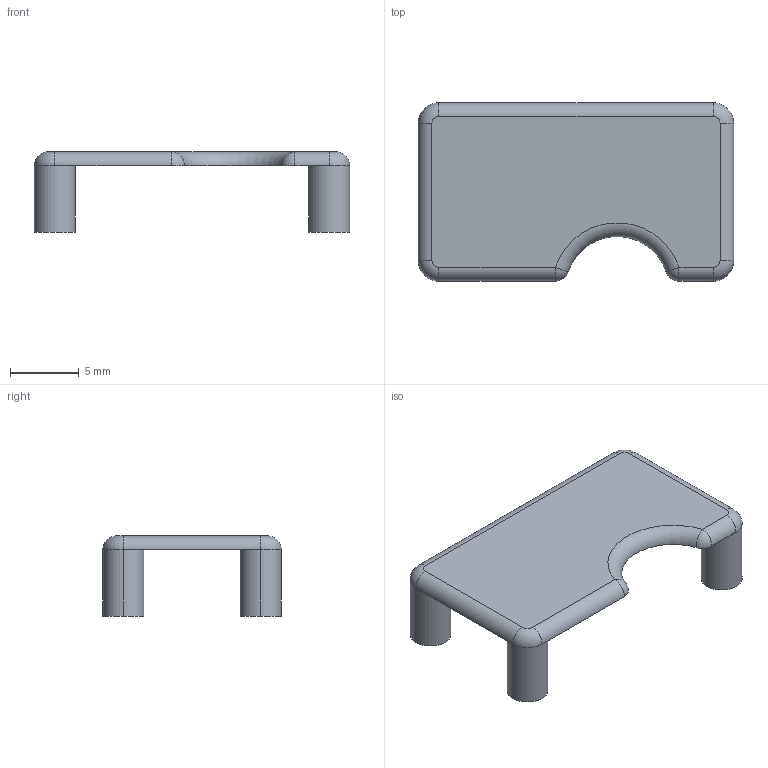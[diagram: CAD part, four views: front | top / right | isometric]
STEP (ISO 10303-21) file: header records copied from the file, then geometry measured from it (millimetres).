
FILE_DESCRIPTION (( 'STEP AP214' ), '1' );
FILE_NAME ('Mag_Release_Cover.step', '2014-05-14T06:09:11', ( 'WarFairy' ), ( '' ), 'SwSTEP 2.0', 'SolidWorks 2013', '' );
FILE_SCHEMA (( 'AUTOMOTIVE_DESIGN' ));
Length unit declared in the file: inch
Products named in the file (1): Mag_Release_Cover
Bounding box: 23 x 13 x 5.85 mm (x, y, z)
Volume: 366.1 mm3; surface area: 734.9 mm2
Topology: 1 solids, 1 shells, 23 faces, 54 edges, 31 vertices
Faces by surface type: cylinder 11, plane 5, torus 5, sphere 2
Entity records: 694 total; most frequent: DIRECTION 136, CARTESIAN_POINT 107, ORIENTED_EDGE 104, AXIS2_PLACEMENT_3D 60, EDGE_CURVE 52, CIRCLE 36, VERTEX_POINT 31, ADVANCED_FACE 23
